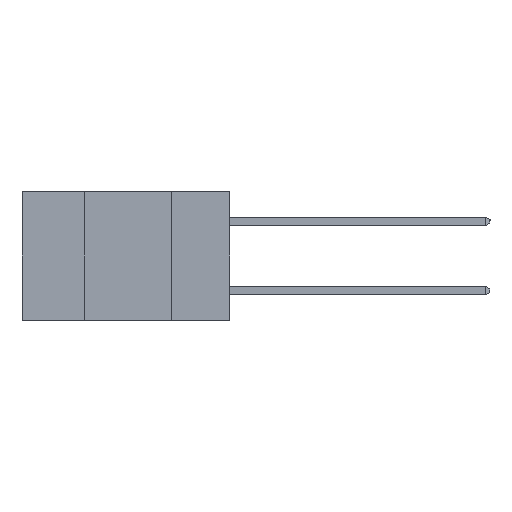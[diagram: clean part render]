
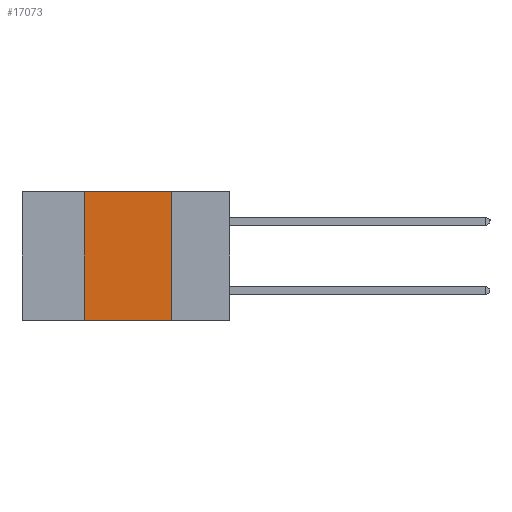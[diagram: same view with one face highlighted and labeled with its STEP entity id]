
A CAD part, left-side view. The second image highlights one B-rep face of the part: STEP entity #17073.
In plain terms, the highlighted planar face has unit normal (-1, 0, 0).
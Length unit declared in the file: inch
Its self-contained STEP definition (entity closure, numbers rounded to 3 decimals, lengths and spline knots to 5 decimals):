
#2423 = EDGE_LOOP ( 'NONE', ( #19933, #6623, #9370, #11685 ) ) ;
#2436 = FACE_OUTER_BOUND ( 'NONE', #2423, .T. ) ;
#2979 = VERTEX_POINT ( 'NONE', #17077 ) ;
#3077 = CARTESIAN_POINT ( 'NONE',  ( 0., 0.6, 0. ) ) ;
#3199 = DIRECTION ( 'NONE',  ( 0., -1., 0. ) ) ;
#4092 = VERTEX_POINT ( 'NONE', #11127 ) ;
#5726 = EDGE_CURVE ( 'NONE', #8224, #4092, #12768, .T. ) ;
#6239 = LINE ( 'NONE', #14348, #6535 ) ;
#6535 = VECTOR ( 'NONE', #20860, 39.37008 ) ;
#6623 = ORIENTED_EDGE ( 'NONE', *, *, #8700, .F. ) ;
#7206 = DIRECTION ( 'NONE',  ( 0., 0., -1. ) ) ;
#8224 = VERTEX_POINT ( 'NONE', #13879 ) ;
#8700 = EDGE_CURVE ( 'NONE', #2979, #20823, #11169, .T. ) ;
#9125 = DIRECTION ( 'NONE',  ( 0., 0., -1. ) ) ;
#9370 = ORIENTED_EDGE ( 'NONE', *, *, #14240, .F. ) ;
#11043 = LINE ( 'NONE', #13819, #11836 ) ;
#11127 = CARTESIAN_POINT ( 'NONE',  ( 0., 0.17, -0.37 ) ) ;
#11169 = LINE ( 'NONE', #3077, #14264 ) ;
#11685 = ORIENTED_EDGE ( 'NONE', *, *, #5726, .T. ) ;
#11836 = VECTOR ( 'NONE', #9125, 39.37008 ) ;
#12020 = PLANE ( 'NONE',  #17869 ) ;
#12350 = VECTOR ( 'NONE', #3199, 39.37008 ) ;
#12768 = LINE ( 'NONE', #19286, #12350 ) ;
#12863 = DIRECTION ( 'NONE',  ( 0., -1., 0. ) ) ;
#13819 = CARTESIAN_POINT ( 'NONE',  ( 0., 0.17, -0.37 ) ) ;
#13879 = CARTESIAN_POINT ( 'NONE',  ( 0., 0.42, -0.37 ) ) ;
#14240 = EDGE_CURVE ( 'NONE', #8224, #2979, #6239, .T. ) ;
#14264 = VECTOR ( 'NONE', #12863, 39.37008 ) ;
#14348 = CARTESIAN_POINT ( 'NONE',  ( 0., 0.42, -0.37 ) ) ;
#16917 = DIRECTION ( 'NONE',  ( 1., 0., 0. ) ) ;
#17073 = ADVANCED_FACE ( 'NONE', ( #2436 ), #12020, .F. ) ;
#17077 = CARTESIAN_POINT ( 'NONE',  ( 0., 0.42, 0. ) ) ;
#17869 = AXIS2_PLACEMENT_3D ( 'NONE', #18538, #16917, #7206 ) ;
#18538 = CARTESIAN_POINT ( 'NONE',  ( 0., 0.6, 0. ) ) ;
#18800 = CARTESIAN_POINT ( 'NONE',  ( 0., 0.17, 0. ) ) ;
#19286 = CARTESIAN_POINT ( 'NONE',  ( 0., 0.6, -0.37 ) ) ;
#19828 = EDGE_CURVE ( 'NONE', #20823, #4092, #11043, .T. ) ;
#19933 = ORIENTED_EDGE ( 'NONE', *, *, #19828, .F. ) ;
#20823 = VERTEX_POINT ( 'NONE', #18800 ) ;
#20860 = DIRECTION ( 'NONE',  ( 0., 0., 1. ) ) ;
